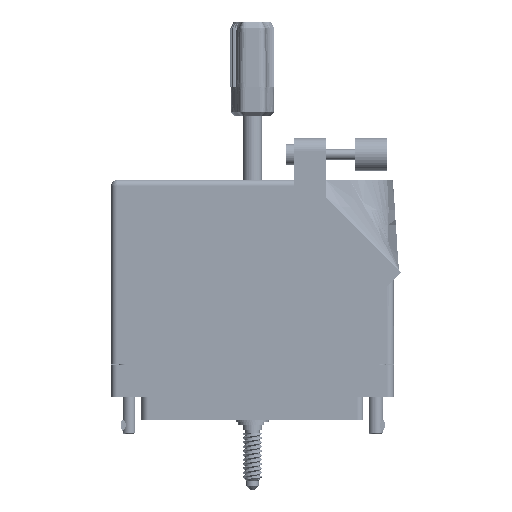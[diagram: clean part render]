
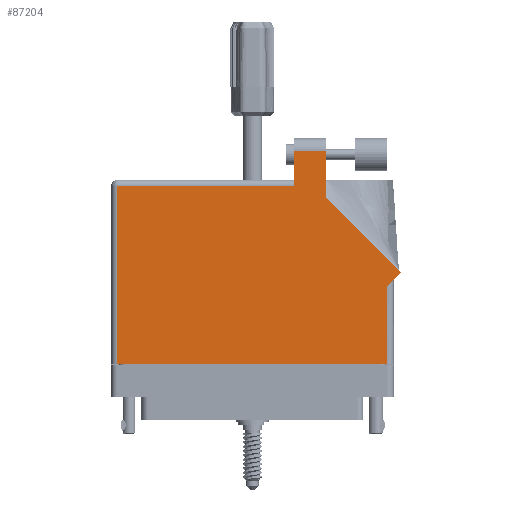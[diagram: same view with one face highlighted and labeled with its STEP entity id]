
A CAD part, front view. The second image highlights one B-rep face of the part: STEP entity #87204.
In plain terms, the highlighted face is planar.
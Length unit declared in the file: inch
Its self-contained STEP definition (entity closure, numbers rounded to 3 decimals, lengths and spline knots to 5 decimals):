
#148 = LINE ( 'NONE', #88790, #94991 ) ;
#2908 = CARTESIAN_POINT ( 'NONE',  ( 0.399, 1.613, 0.617 ) ) ;
#3230 = CARTESIAN_POINT ( 'NONE',  ( 0.399, 1.95, 0.617 ) ) ;
#3770 = VECTOR ( 'NONE', #17556, 39.37008 ) ;
#4165 = VERTEX_POINT ( 'NONE', #82626 ) ;
#6392 = PLANE ( 'NONE',  #36659 ) ;
#6635 = EDGE_CURVE ( 'NONE', #52696, #50178, #31237, .T. ) ;
#7387 = LINE ( 'NONE', #9137, #84565 ) ;
#9137 = CARTESIAN_POINT ( 'NONE',  ( 0.399, 1.95, 0.617 ) ) ;
#9729 = EDGE_CURVE ( 'NONE', #11090, #34014, #35494, .T. ) ;
#11090 = VERTEX_POINT ( 'NONE', #2908 ) ;
#11327 = VECTOR ( 'NONE', #70000, 39.37008 ) ;
#12908 = CARTESIAN_POINT ( 'NONE',  ( -1.359, -0.1, 0.617 ) ) ;
#12960 = VERTEX_POINT ( 'NONE', #52694 ) ;
#12971 = ORIENTED_EDGE ( 'NONE', *, *, #62901, .T. ) ;
#13949 = CARTESIAN_POINT ( 'NONE',  ( 1.297, 0.653, 0.617 ) ) ;
#16705 = CARTESIAN_POINT ( 'NONE',  ( 1.42971, 0.78571, 0.617 ) ) ;
#17556 = DIRECTION ( 'NONE',  ( 0., -1., 0. ) ) ;
#21327 = LINE ( 'NONE', #92096, #3770 ) ;
#21957 = CARTESIAN_POINT ( 'NONE',  ( -1.359, 1.613, 0.617 ) ) ;
#22073 = DIRECTION ( 'NONE',  ( -1., 0., 0. ) ) ;
#25808 = VECTOR ( 'NONE', #83874, 39.37008 ) ;
#28552 = FACE_OUTER_BOUND ( 'NONE', #32091, .T. ) ;
#29532 = ORIENTED_EDGE ( 'NONE', *, *, #88804, .T. ) ;
#29956 = DIRECTION ( 'NONE',  ( 0., 0., -1. ) ) ;
#31237 = LINE ( 'NONE', #16705, #11327 ) ;
#32091 = EDGE_LOOP ( 'NONE', ( #74037, #58186, #57950, #48847, #34867, #12971, #78825, #29532, #71837 ) ) ;
#32959 = DIRECTION ( 'NONE',  ( 0., 1., 0. ) ) ;
#33222 = VERTEX_POINT ( 'NONE', #13949 ) ;
#34014 = VERTEX_POINT ( 'NONE', #63899 ) ;
#34867 = ORIENTED_EDGE ( 'NONE', *, *, #41153, .T. ) ;
#35494 = LINE ( 'NONE', #21957, #45857 ) ;
#35500 = DIRECTION ( 'NONE',  ( 1., 0., 0. ) ) ;
#36659 = AXIS2_PLACEMENT_3D ( 'NONE', #73734, #29956, #22073 ) ;
#39413 = CARTESIAN_POINT ( 'NONE',  ( 1.297, 0.715, 0.617 ) ) ;
#40039 = VECTOR ( 'NONE', #77373, 39.37008 ) ;
#41153 = EDGE_CURVE ( 'NONE', #34014, #4165, #75085, .T. ) ;
#42149 = LINE ( 'NONE', #39413, #25808 ) ;
#44540 = DIRECTION ( 'NONE',  ( -1., 0., 0. ) ) ;
#45857 = VECTOR ( 'NONE', #44540, 39.37008 ) ;
#48847 = ORIENTED_EDGE ( 'NONE', *, *, #9729, .T. ) ;
#50178 = VERTEX_POINT ( 'NONE', #64738 ) ;
#52694 = CARTESIAN_POINT ( 'NONE',  ( 1.297, -0.1, 0.617 ) ) ;
#52696 = VERTEX_POINT ( 'NONE', #66678 ) ;
#53532 = CARTESIAN_POINT ( 'NONE',  ( -1.297, -0.1, 0.617 ) ) ;
#53865 = VERTEX_POINT ( 'NONE', #3230 ) ;
#55416 = CARTESIAN_POINT ( 'NONE',  ( 0.706, 1.50942, 0.617 ) ) ;
#57322 = EDGE_CURVE ( 'NONE', #89754, #53865, #7387, .T. ) ;
#57950 = ORIENTED_EDGE ( 'NONE', *, *, #88546, .T. ) ;
#58043 = DIRECTION ( 'NONE',  ( 0.707, 0.707, 0. ) ) ;
#58186 = ORIENTED_EDGE ( 'NONE', *, *, #57322, .T. ) ;
#58983 = EDGE_CURVE ( 'NONE', #12960, #33222, #42149, .T. ) ;
#59739 = VECTOR ( 'NONE', #32959, 39.37008 ) ;
#61426 = DIRECTION ( 'NONE',  ( -1., 0., 0. ) ) ;
#62901 = EDGE_CURVE ( 'NONE', #4165, #12960, #90495, .T. ) ;
#63899 = CARTESIAN_POINT ( 'NONE',  ( -1.297, 1.613, 0.617 ) ) ;
#64738 = CARTESIAN_POINT ( 'NONE',  ( 0.706, 1.50942, 0.617 ) ) ;
#66678 = CARTESIAN_POINT ( 'NONE',  ( 1.42971, 0.78571, 0.617 ) ) ;
#68203 = VECTOR ( 'NONE', #35500, 39.37008 ) ;
#70000 = DIRECTION ( 'NONE',  ( -0.707, 0.707, 0. ) ) ;
#71837 = ORIENTED_EDGE ( 'NONE', *, *, #6635, .T. ) ;
#73734 = CARTESIAN_POINT ( 'NONE',  ( -1.359, 1.675, 0.617 ) ) ;
#74037 = ORIENTED_EDGE ( 'NONE', *, *, #90047, .T. ) ;
#75085 = LINE ( 'NONE', #53532, #40039 ) ;
#77373 = DIRECTION ( 'NONE',  ( 0., -1., 0. ) ) ;
#78825 = ORIENTED_EDGE ( 'NONE', *, *, #58983, .T. ) ;
#79686 = LINE ( 'NONE', #55416, #59739 ) ;
#82626 = CARTESIAN_POINT ( 'NONE',  ( -1.297, -0.1, 0.617 ) ) ;
#83874 = DIRECTION ( 'NONE',  ( 0., 1., 0. ) ) ;
#84565 = VECTOR ( 'NONE', #61426, 39.37008 ) ;
#87204 = ADVANCED_FACE ( 'NONE', ( #28552 ), #6392, .F. ) ;
#88546 = EDGE_CURVE ( 'NONE', #53865, #11090, #21327, .T. ) ;
#88790 = CARTESIAN_POINT ( 'NONE',  ( 1.359, 0.715, 0.617 ) ) ;
#88804 = EDGE_CURVE ( 'NONE', #33222, #52696, #148, .T. ) ;
#89754 = VERTEX_POINT ( 'NONE', #90475 ) ;
#90047 = EDGE_CURVE ( 'NONE', #50178, #89754, #79686, .T. ) ;
#90475 = CARTESIAN_POINT ( 'NONE',  ( 0.706, 1.95, 0.617 ) ) ;
#90495 = LINE ( 'NONE', #12908, #68203 ) ;
#92096 = CARTESIAN_POINT ( 'NONE',  ( 0.399, 1.675, 0.617 ) ) ;
#94991 = VECTOR ( 'NONE', #58043, 39.37008 ) ;
